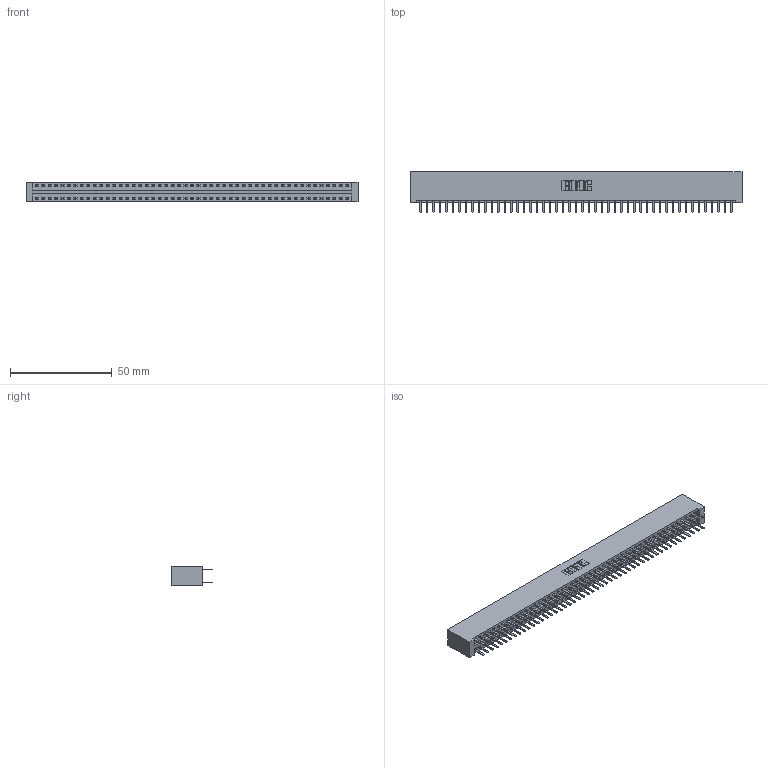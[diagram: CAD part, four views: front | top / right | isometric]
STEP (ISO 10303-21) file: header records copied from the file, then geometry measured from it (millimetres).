
FILE_DESCRIPTION (( 'STEP AP203' ), '1' );
FILE_NAME ('396-098-520-201.STEP', '2019-10-31T04:31:49', ( '' ), ( '' ), 'SwSTEP 2.0', 'SolidWorks 2016', '' );
FILE_SCHEMA (( 'CONFIG_CONTROL_DESIGN' ));
Length unit declared in the file: inch
Products named in the file (3): 345-292-001_345-293-120; 396-098-520-201; 346 Part_No Mounting Lugs
Assembly tree (99 placements, depth 2):
  396-098-520-201
    346 Part_No Mounting Lugs
    345-292-001_345-293-120  x98
Bounding box: 162.81 x 20.02 x 9.4 mm (x, y, z)
Volume: 16461 mm3; surface area: 22799 mm2
Topology: 99 solids, 99 shells, 5602 faces, 16279 edges, 10590 vertices
Faces by surface type: plane 3698, cylinder 1904
Entity records: 30873 total; most frequent: CARTESIAN_POINT 5088, ORIENTED_EDGE 5010, DIRECTION 4517, EDGE_CURVE 2505, VECTOR 2181, LINE 2181, VERTEX_POINT 1666, AXIS2_PLACEMENT_3D 1168
